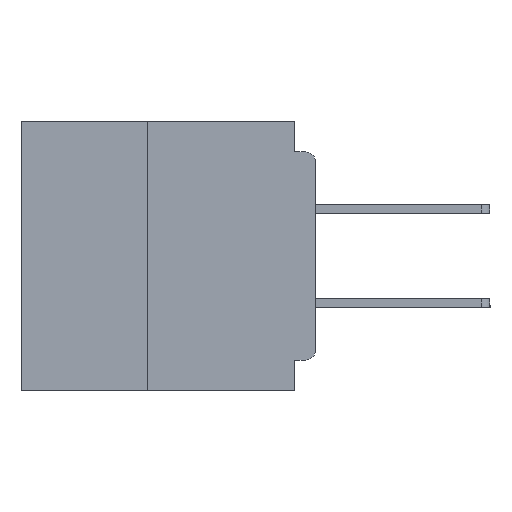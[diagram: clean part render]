
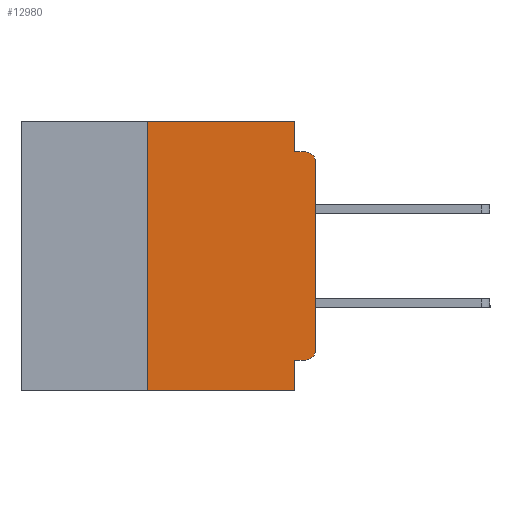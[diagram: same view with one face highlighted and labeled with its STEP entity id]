
A CAD part, left-side view. The second image highlights one B-rep face of the part: STEP entity #12980.
In plain terms, the highlighted planar face has unit normal (-1, 0, 0).
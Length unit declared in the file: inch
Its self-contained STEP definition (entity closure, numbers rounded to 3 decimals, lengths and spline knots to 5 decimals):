
#125 = CARTESIAN_POINT ( 'NONE',  ( 0., 0., -0.34 ) ) ;
#271 = CARTESIAN_POINT ( 'NONE',  ( 0., 0.031, 0. ) ) ;
#870 = CARTESIAN_POINT ( 'NONE',  ( 0., 0.437, 0. ) ) ;
#983 = CARTESIAN_POINT ( 'NONE',  ( 0., 0.437, 0. ) ) ;
#1417 = LINE ( 'NONE', #271, #16377 ) ;
#2685 = DIRECTION ( 'NONE',  ( 0., -1., 0. ) ) ;
#3597 = CARTESIAN_POINT ( 'NONE',  ( 0., 0., 0. ) ) ;
#4834 = CARTESIAN_POINT ( 'NONE',  ( 0., 0.015, -0.06 ) ) ;
#5014 = EDGE_CURVE ( 'NONE', #22301, #34321, #1417, .T. ) ;
#5034 = VERTEX_POINT ( 'NONE', #29845 ) ;
#6115 = EDGE_CURVE ( 'NONE', #34086, #29849, #7186, .T. ) ;
#6222 = ORIENTED_EDGE ( 'NONE', *, *, #5014, .F. ) ;
#6841 = CARTESIAN_POINT ( 'NONE',  ( 0., 0.25, -0.4 ) ) ;
#7186 = LINE ( 'NONE', #25899, #29503 ) ;
#7895 = DIRECTION ( 'NONE',  ( 0., 0., -1. ) ) ;
#8055 = CIRCLE ( 'NONE', #26661, 0.015 ) ;
#8335 = DIRECTION ( 'NONE',  ( 0., 1., 0. ) ) ;
#8617 = CARTESIAN_POINT ( 'NONE',  ( 0., 0., -0.045 ) ) ;
#9152 = CARTESIAN_POINT ( 'NONE',  ( 0., 0.015, -0.34 ) ) ;
#10722 = ORIENTED_EDGE ( 'NONE', *, *, #25718, .T. ) ;
#11009 = CARTESIAN_POINT ( 'NONE',  ( 0., 0.031, -0.355 ) ) ;
#11012 = ORIENTED_EDGE ( 'NONE', *, *, #24269, .T. ) ;
#11043 = ORIENTED_EDGE ( 'NONE', *, *, #23434, .F. ) ;
#11136 = LINE ( 'NONE', #8617, #17983 ) ;
#11194 = CARTESIAN_POINT ( 'NONE',  ( 0., 0.25, 0. ) ) ;
#11444 = LINE ( 'NONE', #29572, #12347 ) ;
#11538 = DIRECTION ( 'NONE',  ( 0., -1., 0. ) ) ;
#11909 = CARTESIAN_POINT ( 'NONE',  ( 0., 0.015, -0.355 ) ) ;
#12072 = DIRECTION ( 'NONE',  ( 0., 0., -1. ) ) ;
#12176 = DIRECTION ( 'NONE',  ( 0., 0., -1. ) ) ;
#12347 = VECTOR ( 'NONE', #12176, 39.37008 ) ;
#12677 = ORIENTED_EDGE ( 'NONE', *, *, #35012, .F. ) ;
#12980 = ADVANCED_FACE ( 'NONE', ( #15882 ), #21659, .F. ) ;
#14059 = VECTOR ( 'NONE', #15929, 39.37008 ) ;
#14071 = VECTOR ( 'NONE', #18334, 39.37008 ) ;
#14800 = EDGE_CURVE ( 'NONE', #21190, #22301, #21817, .T. ) ;
#15882 = FACE_OUTER_BOUND ( 'NONE', #35481, .T. ) ;
#15929 = DIRECTION ( 'NONE',  ( 0., -1., 0. ) ) ;
#16204 = CARTESIAN_POINT ( 'NONE',  ( 0., 0.031, 0. ) ) ;
#16377 = VECTOR ( 'NONE', #21119, 39.37008 ) ;
#16851 = ORIENTED_EDGE ( 'NONE', *, *, #33396, .T. ) ;
#17591 = CARTESIAN_POINT ( 'NONE',  ( 0., 0.25, -0.4 ) ) ;
#17983 = VECTOR ( 'NONE', #11538, 39.37008 ) ;
#18123 = LINE ( 'NONE', #20413, #24954 ) ;
#18334 = DIRECTION ( 'NONE',  ( 0., 0., 1. ) ) ;
#18643 = EDGE_CURVE ( 'NONE', #34321, #22735, #11136, .T. ) ;
#18859 = DIRECTION ( 'NONE',  ( 0., 0., -1. ) ) ;
#20413 = CARTESIAN_POINT ( 'NONE',  ( 0., 0.437, -0.4 ) ) ;
#21119 = DIRECTION ( 'NONE',  ( 0., 0., -1. ) ) ;
#21190 = VERTEX_POINT ( 'NONE', #11194 ) ;
#21374 = AXIS2_PLACEMENT_3D ( 'NONE', #870, #36143, #18859 ) ;
#21446 = VERTEX_POINT ( 'NONE', #125 ) ;
#21528 = DIRECTION ( 'NONE',  ( 0., 0., 1. ) ) ;
#21659 = PLANE ( 'NONE',  #21374 ) ;
#21817 = LINE ( 'NONE', #983, #14059 ) ;
#21831 = LINE ( 'NONE', #3597, #14071 ) ;
#22301 = VERTEX_POINT ( 'NONE', #16204 ) ;
#22690 = VERTEX_POINT ( 'NONE', #17591 ) ;
#22735 = VERTEX_POINT ( 'NONE', #29372 ) ;
#23434 = EDGE_CURVE ( 'NONE', #29849, #5034, #11444, .T. ) ;
#24269 = EDGE_CURVE ( 'NONE', #21446, #35595, #21831, .T. ) ;
#24954 = VECTOR ( 'NONE', #2685, 39.37008 ) ;
#25358 = DIRECTION ( 'NONE',  ( -1., 0., 0. ) ) ;
#25384 = EDGE_CURVE ( 'NONE', #22690, #5034, #18123, .T. ) ;
#25718 = EDGE_CURVE ( 'NONE', #35595, #22735, #8055, .T. ) ;
#25899 = CARTESIAN_POINT ( 'NONE',  ( 0., 0., -0.355 ) ) ;
#26661 = AXIS2_PLACEMENT_3D ( 'NONE', #4834, #25358, #7895 ) ;
#28810 = ORIENTED_EDGE ( 'NONE', *, *, #25384, .T. ) ;
#29372 = CARTESIAN_POINT ( 'NONE',  ( 0., 0.015, -0.045 ) ) ;
#29478 = DIRECTION ( 'NONE',  ( -1., 0., 0. ) ) ;
#29503 = VECTOR ( 'NONE', #8335, 39.37008 ) ;
#29572 = CARTESIAN_POINT ( 'NONE',  ( 0., 0.031, -0.4 ) ) ;
#29591 = CARTESIAN_POINT ( 'NONE',  ( 0., 0., -0.06 ) ) ;
#29776 = ORIENTED_EDGE ( 'NONE', *, *, #14800, .F. ) ;
#29793 = VECTOR ( 'NONE', #21528, 39.37008 ) ;
#29845 = CARTESIAN_POINT ( 'NONE',  ( 0., 0.031, -0.4 ) ) ;
#29849 = VERTEX_POINT ( 'NONE', #11009 ) ;
#33058 = CARTESIAN_POINT ( 'NONE',  ( 0., 0.031, -0.045 ) ) ;
#33396 = EDGE_CURVE ( 'NONE', #34086, #21446, #35681, .T. ) ;
#34086 = VERTEX_POINT ( 'NONE', #11909 ) ;
#34321 = VERTEX_POINT ( 'NONE', #33058 ) ;
#34809 = ORIENTED_EDGE ( 'NONE', *, *, #18643, .F. ) ;
#35012 = EDGE_CURVE ( 'NONE', #22690, #21190, #37413, .T. ) ;
#35109 = ORIENTED_EDGE ( 'NONE', *, *, #6115, .F. ) ;
#35481 = EDGE_LOOP ( 'NONE', ( #11012, #10722, #34809, #6222, #29776, #12677, #28810, #11043, #35109, #16851 ) ) ;
#35595 = VERTEX_POINT ( 'NONE', #29591 ) ;
#35681 = CIRCLE ( 'NONE', #36188, 0.015 ) ;
#36143 = DIRECTION ( 'NONE',  ( 1., 0., 0. ) ) ;
#36188 = AXIS2_PLACEMENT_3D ( 'NONE', #9152, #29478, #12072 ) ;
#37413 = LINE ( 'NONE', #6841, #29793 ) ;
